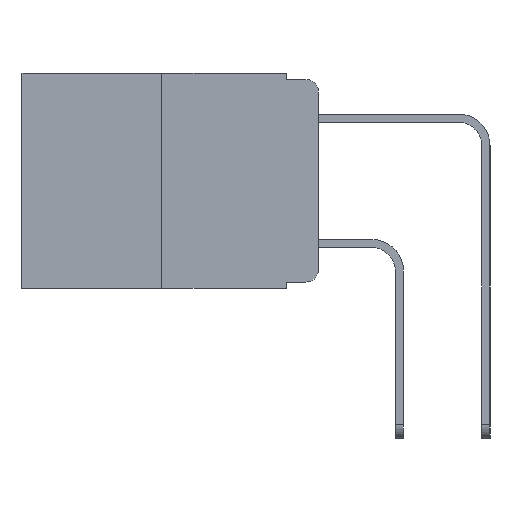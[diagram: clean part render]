
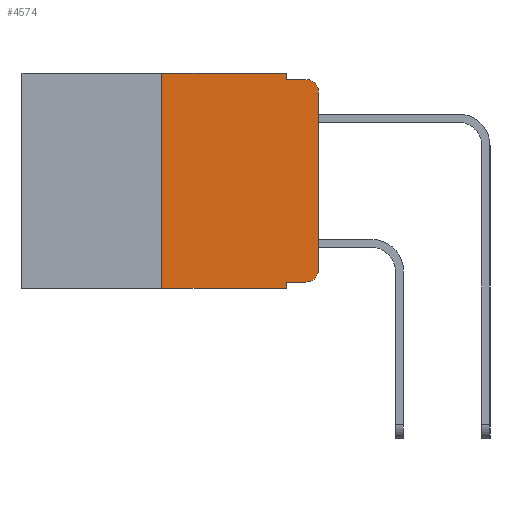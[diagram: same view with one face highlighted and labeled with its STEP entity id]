
A CAD part, left-side view. The second image highlights one B-rep face of the part: STEP entity #4574.
In plain terms, the highlighted planar face has unit normal (-1, 0, 0).
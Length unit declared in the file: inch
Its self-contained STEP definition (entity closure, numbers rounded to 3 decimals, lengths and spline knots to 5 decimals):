
#124 = EDGE_CURVE ( 'NONE', #18531, #12765, #1053, .T. ) ;
#214 = VERTEX_POINT ( 'NONE', #13933 ) ;
#357 = EDGE_CURVE ( 'NONE', #18531, #15540, #6339, .T. ) ;
#638 = CARTESIAN_POINT ( 'NONE',  ( 0., 0.02, -0.03 ) ) ;
#649 = VERTEX_POINT ( 'NONE', #13910 ) ;
#677 = CARTESIAN_POINT ( 'NONE',  ( 0., 0.051, -0.343 ) ) ;
#729 = CARTESIAN_POINT ( 'NONE',  ( 0., 0., 0. ) ) ;
#1053 = LINE ( 'NONE', #8532, #12479 ) ;
#1066 = CARTESIAN_POINT ( 'NONE',  ( 0., 0.25, 0. ) ) ;
#1347 = DIRECTION ( 'NONE',  ( -1., 0., 0. ) ) ;
#1417 = ORIENTED_EDGE ( 'NONE', *, *, #16733, .T. ) ;
#1636 = EDGE_CURVE ( 'NONE', #2970, #2315, #8303, .T. ) ;
#1706 = VECTOR ( 'NONE', #3160, 39.37008 ) ;
#1947 = VERTEX_POINT ( 'NONE', #11179 ) ;
#2315 = VERTEX_POINT ( 'NONE', #16229 ) ;
#2652 = LINE ( 'NONE', #17080, #17578 ) ;
#2772 = ORIENTED_EDGE ( 'NONE', *, *, #5465, .T. ) ;
#2970 = VERTEX_POINT ( 'NONE', #3747 ) ;
#3046 = DIRECTION ( 'NONE',  ( -1., 0., 0. ) ) ;
#3060 = ORIENTED_EDGE ( 'NONE', *, *, #3459, .F. ) ;
#3130 = VERTEX_POINT ( 'NONE', #13367 ) ;
#3160 = DIRECTION ( 'NONE',  ( 0., -1., 0. ) ) ;
#3459 = EDGE_CURVE ( 'NONE', #14636, #2970, #5068, .T. ) ;
#3747 = CARTESIAN_POINT ( 'NONE',  ( 0., 0.051, 0. ) ) ;
#3977 = EDGE_CURVE ( 'NONE', #649, #214, #17229, .T. ) ;
#4138 = DIRECTION ( 'NONE',  ( 0., 0., -1. ) ) ;
#4156 = CARTESIAN_POINT ( 'NONE',  ( 0., 0.051, 0. ) ) ;
#4574 = ADVANCED_FACE ( 'NONE', ( #5618 ), #17513, .F. ) ;
#5068 = LINE ( 'NONE', #12780, #14926 ) ;
#5177 = DIRECTION ( 'NONE',  ( 0., 0., -1. ) ) ;
#5465 = EDGE_CURVE ( 'NONE', #1947, #15540, #2652, .T. ) ;
#5618 = FACE_OUTER_BOUND ( 'NONE', #10451, .T. ) ;
#6195 = EDGE_CURVE ( 'NONE', #1947, #14636, #15527, .T. ) ;
#6285 = ORIENTED_EDGE ( 'NONE', *, *, #1636, .F. ) ;
#6339 = LINE ( 'NONE', #6873, #9330 ) ;
#6866 = DIRECTION ( 'NONE',  ( 0., 0., 1. ) ) ;
#6873 = CARTESIAN_POINT ( 'NONE',  ( 0., 0.051, 0. ) ) ;
#7049 = DIRECTION ( 'NONE',  ( 0., 0., -1. ) ) ;
#7887 = DIRECTION ( 'NONE',  ( 0., -1., 0. ) ) ;
#7947 = CARTESIAN_POINT ( 'NONE',  ( 0., 0.02, -0.333 ) ) ;
#7968 = ORIENTED_EDGE ( 'NONE', *, *, #357, .F. ) ;
#8203 = CARTESIAN_POINT ( 'NONE',  ( 0., 0.473, 0. ) ) ;
#8303 = LINE ( 'NONE', #4156, #11901 ) ;
#8314 = ORIENTED_EDGE ( 'NONE', *, *, #124, .T. ) ;
#8532 = CARTESIAN_POINT ( 'NONE',  ( 0., 0.051, -0.333 ) ) ;
#8737 = CARTESIAN_POINT ( 'NONE',  ( 0., 0.051, -0.333 ) ) ;
#8994 = CIRCLE ( 'NONE', #11247, 0.02 ) ;
#9215 = DIRECTION ( 'NONE',  ( 0., 0., -1. ) ) ;
#9330 = VECTOR ( 'NONE', #7049, 39.37008 ) ;
#9463 = AXIS2_PLACEMENT_3D ( 'NONE', #638, #1347, #9215 ) ;
#9605 = EDGE_CURVE ( 'NONE', #2315, #214, #16450, .T. ) ;
#9945 = ORIENTED_EDGE ( 'NONE', *, *, #9605, .F. ) ;
#10451 = EDGE_LOOP ( 'NONE', ( #1417, #11869, #9945, #6285, #3060, #14586, #2772, #7968, #8314, #10646 ) ) ;
#10567 = CARTESIAN_POINT ( 'NONE',  ( 0., 0.051, -0.01 ) ) ;
#10646 = ORIENTED_EDGE ( 'NONE', *, *, #18069, .T. ) ;
#11179 = CARTESIAN_POINT ( 'NONE',  ( 0., 0.25, -0.343 ) ) ;
#11247 = AXIS2_PLACEMENT_3D ( 'NONE', #11800, #3046, #13182 ) ;
#11364 = DIRECTION ( 'NONE',  ( 0., -1., 0. ) ) ;
#11494 = VECTOR ( 'NONE', #14016, 39.37008 ) ;
#11800 = CARTESIAN_POINT ( 'NONE',  ( 0., 0.02, -0.313 ) ) ;
#11869 = ORIENTED_EDGE ( 'NONE', *, *, #3977, .T. ) ;
#11901 = VECTOR ( 'NONE', #4138, 39.37008 ) ;
#11914 = LINE ( 'NONE', #729, #11494 ) ;
#11989 = VECTOR ( 'NONE', #6866, 39.37008 ) ;
#12479 = VECTOR ( 'NONE', #7887, 39.37008 ) ;
#12765 = VERTEX_POINT ( 'NONE', #7947 ) ;
#12780 = CARTESIAN_POINT ( 'NONE',  ( 0., 0.473, 0. ) ) ;
#13182 = DIRECTION ( 'NONE',  ( 0., 0., -1. ) ) ;
#13367 = CARTESIAN_POINT ( 'NONE',  ( 0., 0., -0.313 ) ) ;
#13661 = DIRECTION ( 'NONE',  ( 1., 0., 0. ) ) ;
#13910 = CARTESIAN_POINT ( 'NONE',  ( 0., 0., -0.03 ) ) ;
#13933 = CARTESIAN_POINT ( 'NONE',  ( 0., 0.02, -0.01 ) ) ;
#14016 = DIRECTION ( 'NONE',  ( 0., 0., 1. ) ) ;
#14586 = ORIENTED_EDGE ( 'NONE', *, *, #6195, .F. ) ;
#14636 = VERTEX_POINT ( 'NONE', #1066 ) ;
#14926 = VECTOR ( 'NONE', #11364, 39.37008 ) ;
#15055 = AXIS2_PLACEMENT_3D ( 'NONE', #8203, #13661, #5177 ) ;
#15527 = LINE ( 'NONE', #16374, #11989 ) ;
#15540 = VERTEX_POINT ( 'NONE', #677 ) ;
#16229 = CARTESIAN_POINT ( 'NONE',  ( 0., 0.051, -0.01 ) ) ;
#16374 = CARTESIAN_POINT ( 'NONE',  ( 0., 0.25, 0. ) ) ;
#16450 = LINE ( 'NONE', #10567, #1706 ) ;
#16733 = EDGE_CURVE ( 'NONE', #3130, #649, #11914, .T. ) ;
#17080 = CARTESIAN_POINT ( 'NONE',  ( 0., 0.473, -0.343 ) ) ;
#17229 = CIRCLE ( 'NONE', #9463, 0.02 ) ;
#17513 = PLANE ( 'NONE',  #15055 ) ;
#17578 = VECTOR ( 'NONE', #18349, 39.37008 ) ;
#18069 = EDGE_CURVE ( 'NONE', #12765, #3130, #8994, .T. ) ;
#18349 = DIRECTION ( 'NONE',  ( 0., -1., 0. ) ) ;
#18531 = VERTEX_POINT ( 'NONE', #8737 ) ;
